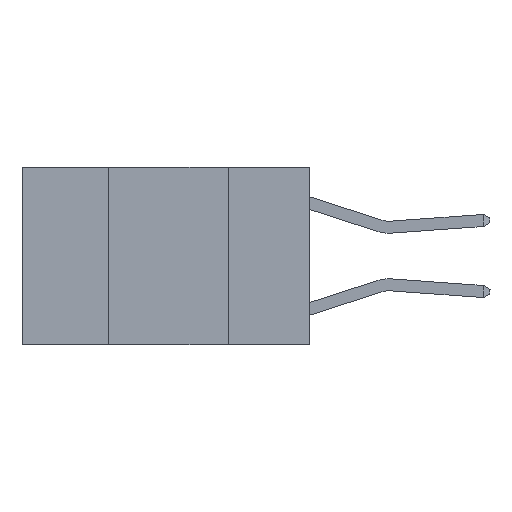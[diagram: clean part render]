
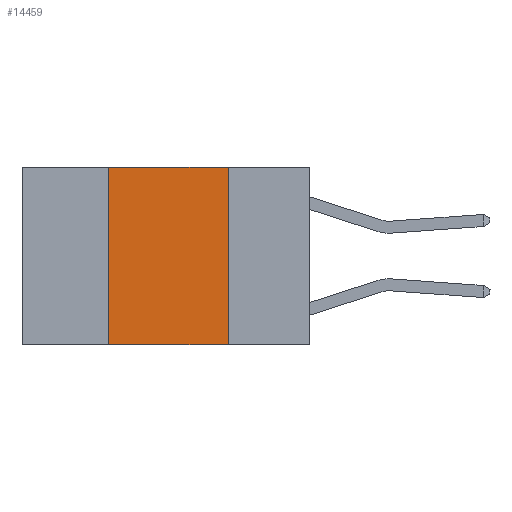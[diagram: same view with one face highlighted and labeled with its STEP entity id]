
A CAD part, left-side view. The second image highlights one B-rep face of the part: STEP entity #14459.
In plain terms, the highlighted planar face has unit normal (-1, 0, 0).
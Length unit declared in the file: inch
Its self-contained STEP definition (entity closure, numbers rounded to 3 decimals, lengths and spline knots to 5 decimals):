
#660 = CARTESIAN_POINT ( 'NONE',  ( 0., 0.17, 0. ) ) ;
#1016 = FACE_OUTER_BOUND ( 'NONE', #6256, .T. ) ;
#2281 = ORIENTED_EDGE ( 'NONE', *, *, #13271, .F. ) ;
#2577 = DIRECTION ( 'NONE',  ( 0., 0., -1. ) ) ;
#2984 = DIRECTION ( 'NONE',  ( 0., -1., 0. ) ) ;
#3552 = EDGE_CURVE ( 'NONE', #7707, #6594, #11686, .T. ) ;
#6081 = CARTESIAN_POINT ( 'NONE',  ( 0., 0.42, 0. ) ) ;
#6179 = CARTESIAN_POINT ( 'NONE',  ( 0., 0.6, -0.37 ) ) ;
#6256 = EDGE_LOOP ( 'NONE', ( #11017, #17991, #2281, #11205 ) ) ;
#6448 = VECTOR ( 'NONE', #2577, 39.37008 ) ;
#6594 = VERTEX_POINT ( 'NONE', #15881 ) ;
#7067 = VERTEX_POINT ( 'NONE', #16453 ) ;
#7123 = CARTESIAN_POINT ( 'NONE',  ( 0., 0.6, 0. ) ) ;
#7527 = CARTESIAN_POINT ( 'NONE',  ( 0., 0.17, 0. ) ) ;
#7604 = CARTESIAN_POINT ( 'NONE',  ( 0., 0.42, 0. ) ) ;
#7707 = VERTEX_POINT ( 'NONE', #7527 ) ;
#7862 = VECTOR ( 'NONE', #18892, 39.37008 ) ;
#9472 = EDGE_CURVE ( 'NONE', #10886, #7707, #14271, .T. ) ;
#9557 = VECTOR ( 'NONE', #12179, 39.37008 ) ;
#9825 = PLANE ( 'NONE',  #18812 ) ;
#10598 = CARTESIAN_POINT ( 'NONE',  ( 0., 0.6, 0. ) ) ;
#10886 = VERTEX_POINT ( 'NONE', #7604 ) ;
#11017 = ORIENTED_EDGE ( 'NONE', *, *, #3552, .F. ) ;
#11205 = ORIENTED_EDGE ( 'NONE', *, *, #13247, .T. ) ;
#11686 = LINE ( 'NONE', #660, #6448 ) ;
#12179 = DIRECTION ( 'NONE',  ( 0., 0., 1. ) ) ;
#13223 = DIRECTION ( 'NONE',  ( 1., 0., 0. ) ) ;
#13247 = EDGE_CURVE ( 'NONE', #7067, #6594, #16686, .T. ) ;
#13271 = EDGE_CURVE ( 'NONE', #7067, #10886, #18494, .T. ) ;
#14271 = LINE ( 'NONE', #10598, #7862 ) ;
#14459 = ADVANCED_FACE ( 'NONE', ( #1016 ), #9825, .F. ) ;
#14827 = DIRECTION ( 'NONE',  ( 0., 0., -1. ) ) ;
#14987 = VECTOR ( 'NONE', #2984, 39.37008 ) ;
#15881 = CARTESIAN_POINT ( 'NONE',  ( 0., 0.17, -0.37 ) ) ;
#16453 = CARTESIAN_POINT ( 'NONE',  ( 0., 0.42, -0.37 ) ) ;
#16686 = LINE ( 'NONE', #6179, #14987 ) ;
#17991 = ORIENTED_EDGE ( 'NONE', *, *, #9472, .F. ) ;
#18494 = LINE ( 'NONE', #6081, #9557 ) ;
#18812 = AXIS2_PLACEMENT_3D ( 'NONE', #7123, #13223, #14827 ) ;
#18892 = DIRECTION ( 'NONE',  ( 0., -1., 0. ) ) ;
